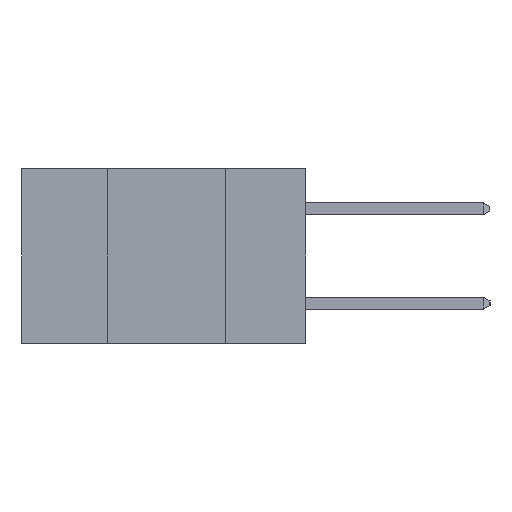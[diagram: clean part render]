
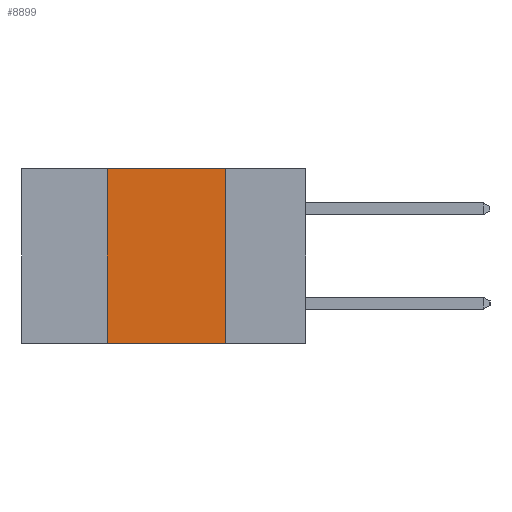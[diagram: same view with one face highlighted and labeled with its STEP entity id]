
A CAD part, left-side view. The second image highlights one B-rep face of the part: STEP entity #8899.
In plain terms, the highlighted planar face has unit normal (-1, 0, 0).
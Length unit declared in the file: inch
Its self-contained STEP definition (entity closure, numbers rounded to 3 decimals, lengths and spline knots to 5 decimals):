
#1830 = DIRECTION ( 'NONE',  ( 1., 0., 0. ) ) ;
#2201 = VECTOR ( 'NONE', #15617, 39.37008 ) ;
#2465 = CARTESIAN_POINT ( 'NONE',  ( 0., 0.6, -0.37 ) ) ;
#3413 = ORIENTED_EDGE ( 'NONE', *, *, #14640, .F. ) ;
#4064 = CARTESIAN_POINT ( 'NONE',  ( 0., 0.42, -0.37 ) ) ;
#5657 = CARTESIAN_POINT ( 'NONE',  ( 0., 0.42, 0. ) ) ;
#5914 = VERTEX_POINT ( 'NONE', #13986 ) ;
#6853 = LINE ( 'NONE', #16103, #15051 ) ;
#7010 = CARTESIAN_POINT ( 'NONE',  ( 0., 0.6, 0. ) ) ;
#7363 = DIRECTION ( 'NONE',  ( 0., 0., 1. ) ) ;
#7373 = ORIENTED_EDGE ( 'NONE', *, *, #14426, .T. ) ;
#8421 = PLANE ( 'NONE',  #17554 ) ;
#8532 = CARTESIAN_POINT ( 'NONE',  ( 0., 0.42, -0.37 ) ) ;
#8899 = ADVANCED_FACE ( 'NONE', ( #12057 ), #8421, .F. ) ;
#10114 = CARTESIAN_POINT ( 'NONE',  ( 0., 0.6, 0. ) ) ;
#11529 = EDGE_CURVE ( 'NONE', #14380, #5914, #19509, .T. ) ;
#11687 = EDGE_CURVE ( 'NONE', #13428, #14380, #12670, .T. ) ;
#11927 = DIRECTION ( 'NONE',  ( 0., -1., 0. ) ) ;
#12057 = FACE_OUTER_BOUND ( 'NONE', #14337, .T. ) ;
#12545 = VERTEX_POINT ( 'NONE', #19165 ) ;
#12670 = LINE ( 'NONE', #4064, #20755 ) ;
#13376 = DIRECTION ( 'NONE',  ( 0., 0., -1. ) ) ;
#13428 = VERTEX_POINT ( 'NONE', #8532 ) ;
#13986 = CARTESIAN_POINT ( 'NONE',  ( 0., 0.17, 0. ) ) ;
#14337 = EDGE_LOOP ( 'NONE', ( #3413, #18107, #20853, #7373 ) ) ;
#14380 = VERTEX_POINT ( 'NONE', #5657 ) ;
#14426 = EDGE_CURVE ( 'NONE', #13428, #12545, #15823, .T. ) ;
#14640 = EDGE_CURVE ( 'NONE', #5914, #12545, #6853, .T. ) ;
#15051 = VECTOR ( 'NONE', #17721, 39.37008 ) ;
#15198 = VECTOR ( 'NONE', #11927, 39.37008 ) ;
#15617 = DIRECTION ( 'NONE',  ( 0., -1., 0. ) ) ;
#15823 = LINE ( 'NONE', #2465, #2201 ) ;
#16103 = CARTESIAN_POINT ( 'NONE',  ( 0., 0.17, -0.37 ) ) ;
#17554 = AXIS2_PLACEMENT_3D ( 'NONE', #10114, #1830, #13376 ) ;
#17721 = DIRECTION ( 'NONE',  ( 0., 0., -1. ) ) ;
#18107 = ORIENTED_EDGE ( 'NONE', *, *, #11529, .F. ) ;
#19165 = CARTESIAN_POINT ( 'NONE',  ( 0., 0.17, -0.37 ) ) ;
#19509 = LINE ( 'NONE', #7010, #15198 ) ;
#20755 = VECTOR ( 'NONE', #7363, 39.37008 ) ;
#20853 = ORIENTED_EDGE ( 'NONE', *, *, #11687, .F. ) ;
